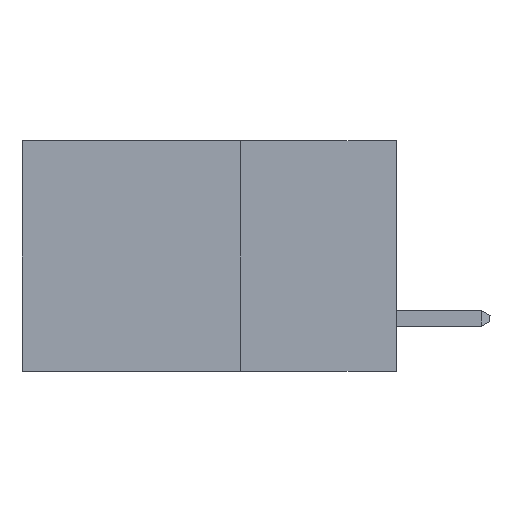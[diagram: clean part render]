
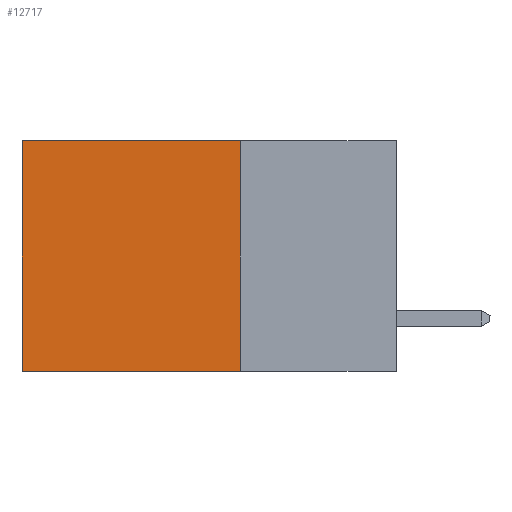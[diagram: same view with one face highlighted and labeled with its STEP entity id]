
A CAD part, left-side view. The second image highlights one B-rep face of the part: STEP entity #12717.
In plain terms, the highlighted planar face has unit normal (-1, 0, 0).
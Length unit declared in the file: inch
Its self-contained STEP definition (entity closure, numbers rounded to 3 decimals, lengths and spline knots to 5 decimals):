
#78 = EDGE_CURVE ( 'NONE', #4881, #4108, #9144, .T. ) ;
#139 = ORIENTED_EDGE ( 'NONE', *, *, #6500, .T. ) ;
#224 = CARTESIAN_POINT ( 'NONE',  ( 0.2615, 0.25, 0. ) ) ;
#569 = CARTESIAN_POINT ( 'NONE',  ( 0.2615, 0.25, -0.37 ) ) ;
#664 = PLANE ( 'NONE',  #3754 ) ;
#1178 = VECTOR ( 'NONE', #3856, 39.37008 ) ;
#1272 = LINE ( 'NONE', #9887, #8590 ) ;
#1349 = VERTEX_POINT ( 'NONE', #224 ) ;
#2025 = VERTEX_POINT ( 'NONE', #7762 ) ;
#2115 = DIRECTION ( 'NONE',  ( 1., 0., 0. ) ) ;
#2962 = EDGE_CURVE ( 'NONE', #1349, #2025, #1272, .T. ) ;
#3663 = CARTESIAN_POINT ( 'NONE',  ( 0.2615, 0.25, -0.37 ) ) ;
#3700 = CARTESIAN_POINT ( 'NONE',  ( 0.2615, 0.6, -0.37 ) ) ;
#3754 = AXIS2_PLACEMENT_3D ( 'NONE', #3663, #2115, #10576 ) ;
#3856 = DIRECTION ( 'NONE',  ( 0., 1., 0. ) ) ;
#4108 = VERTEX_POINT ( 'NONE', #3700 ) ;
#4621 = DIRECTION ( 'NONE',  ( 0., 1., 0. ) ) ;
#4759 = DIRECTION ( 'NONE',  ( 0., 0., -1. ) ) ;
#4881 = VERTEX_POINT ( 'NONE', #569 ) ;
#5570 = EDGE_LOOP ( 'NONE', ( #139, #11435, #7050, #11050 ) ) ;
#6179 = VECTOR ( 'NONE', #4759, 39.37008 ) ;
#6500 = EDGE_CURVE ( 'NONE', #2025, #4108, #9442, .T. ) ;
#7050 = ORIENTED_EDGE ( 'NONE', *, *, #10251, .F. ) ;
#7762 = CARTESIAN_POINT ( 'NONE',  ( 0.2615, 0.6, 0. ) ) ;
#8590 = VECTOR ( 'NONE', #4621, 39.37008 ) ;
#9144 = LINE ( 'NONE', #13387, #1178 ) ;
#9193 = LINE ( 'NONE', #12234, #6179 ) ;
#9442 = LINE ( 'NONE', #13545, #10773 ) ;
#9887 = CARTESIAN_POINT ( 'NONE',  ( 0.2615, 0.25, 0. ) ) ;
#10251 = EDGE_CURVE ( 'NONE', #1349, #4881, #9193, .T. ) ;
#10576 = DIRECTION ( 'NONE',  ( 0., 0., -1. ) ) ;
#10773 = VECTOR ( 'NONE', #13595, 39.37008 ) ;
#11050 = ORIENTED_EDGE ( 'NONE', *, *, #2962, .T. ) ;
#11435 = ORIENTED_EDGE ( 'NONE', *, *, #78, .F. ) ;
#12234 = CARTESIAN_POINT ( 'NONE',  ( 0.2615, 0.25, -0.37 ) ) ;
#12717 = ADVANCED_FACE ( 'NONE', ( #13176 ), #664, .F. ) ;
#13176 = FACE_OUTER_BOUND ( 'NONE', #5570, .T. ) ;
#13387 = CARTESIAN_POINT ( 'NONE',  ( 0.2615, 0.25, -0.37 ) ) ;
#13545 = CARTESIAN_POINT ( 'NONE',  ( 0.2615, 0.6, -0.37 ) ) ;
#13595 = DIRECTION ( 'NONE',  ( 0., 0., -1. ) ) ;
